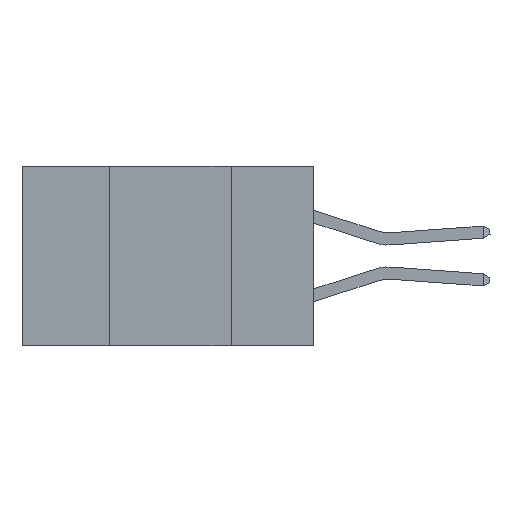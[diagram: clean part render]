
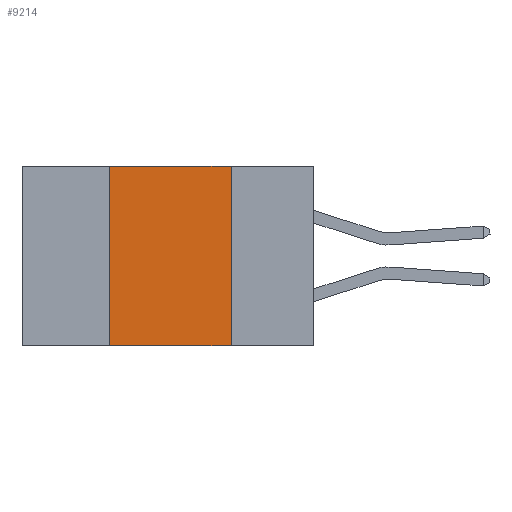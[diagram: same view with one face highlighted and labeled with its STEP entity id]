
A CAD part, left-side view. The second image highlights one B-rep face of the part: STEP entity #9214.
In plain terms, the highlighted planar face has unit normal (-1, 0, 0).
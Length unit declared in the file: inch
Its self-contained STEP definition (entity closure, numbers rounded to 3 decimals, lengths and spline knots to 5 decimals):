
#207 = VERTEX_POINT ( 'NONE', #11212 ) ;
#610 = EDGE_CURVE ( 'NONE', #207, #8759, #2955, .T. ) ;
#1058 = VERTEX_POINT ( 'NONE', #6693 ) ;
#1304 = ORIENTED_EDGE ( 'NONE', *, *, #3100, .F. ) ;
#2170 = EDGE_LOOP ( 'NONE', ( #9764, #9335, #1304, #5371 ) ) ;
#2894 = DIRECTION ( 'NONE',  ( 0., 0., -1. ) ) ;
#2953 = CARTESIAN_POINT ( 'NONE',  ( 0., 0.6, 0. ) ) ;
#2955 = LINE ( 'NONE', #7651, #9782 ) ;
#3100 = EDGE_CURVE ( 'NONE', #1058, #3528, #3128, .T. ) ;
#3128 = LINE ( 'NONE', #7819, #6423 ) ;
#3332 = DIRECTION ( 'NONE',  ( 0., -1., 0. ) ) ;
#3378 = VECTOR ( 'NONE', #3332, 39.37008 ) ;
#3528 = VERTEX_POINT ( 'NONE', #6929 ) ;
#4105 = DIRECTION ( 'NONE',  ( 0., -1., 0. ) ) ;
#5371 = ORIENTED_EDGE ( 'NONE', *, *, #8024, .T. ) ;
#6423 = VECTOR ( 'NONE', #9678, 39.37008 ) ;
#6649 = FACE_OUTER_BOUND ( 'NONE', #2170, .T. ) ;
#6693 = CARTESIAN_POINT ( 'NONE',  ( 0., 0.42, -0.37 ) ) ;
#6929 = CARTESIAN_POINT ( 'NONE',  ( 0., 0.42, 0. ) ) ;
#7286 = CARTESIAN_POINT ( 'NONE',  ( 0., 0.6, 0. ) ) ;
#7350 = LINE ( 'NONE', #7286, #3378 ) ;
#7651 = CARTESIAN_POINT ( 'NONE',  ( 0., 0.17, 0. ) ) ;
#7819 = CARTESIAN_POINT ( 'NONE',  ( 0., 0.42, 0. ) ) ;
#8024 = EDGE_CURVE ( 'NONE', #1058, #8759, #10590, .T. ) ;
#8088 = VECTOR ( 'NONE', #4105, 39.37008 ) ;
#8626 = EDGE_CURVE ( 'NONE', #3528, #207, #7350, .T. ) ;
#8759 = VERTEX_POINT ( 'NONE', #12139 ) ;
#8800 = CARTESIAN_POINT ( 'NONE',  ( 0., 0.6, -0.37 ) ) ;
#9214 = ADVANCED_FACE ( 'NONE', ( #6649 ), #10407, .F. ) ;
#9335 = ORIENTED_EDGE ( 'NONE', *, *, #8626, .F. ) ;
#9678 = DIRECTION ( 'NONE',  ( 0., 0., 1. ) ) ;
#9764 = ORIENTED_EDGE ( 'NONE', *, *, #610, .F. ) ;
#9782 = VECTOR ( 'NONE', #2894, 39.37008 ) ;
#10176 = DIRECTION ( 'NONE',  ( 1., 0., 0. ) ) ;
#10230 = DIRECTION ( 'NONE',  ( 0., 0., -1. ) ) ;
#10407 = PLANE ( 'NONE',  #10478 ) ;
#10478 = AXIS2_PLACEMENT_3D ( 'NONE', #2953, #10176, #10230 ) ;
#10590 = LINE ( 'NONE', #8800, #8088 ) ;
#11212 = CARTESIAN_POINT ( 'NONE',  ( 0., 0.17, 0. ) ) ;
#12139 = CARTESIAN_POINT ( 'NONE',  ( 0., 0.17, -0.37 ) ) ;
